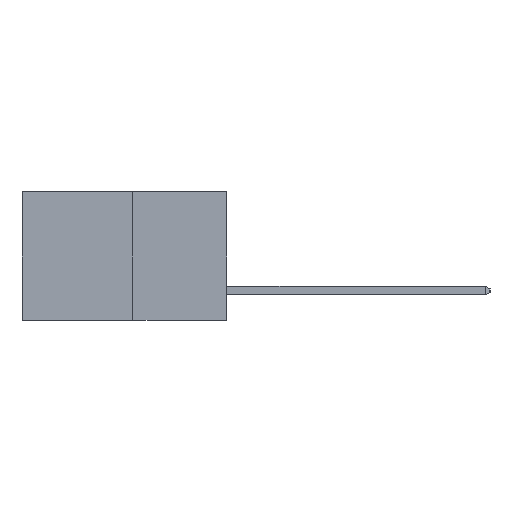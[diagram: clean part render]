
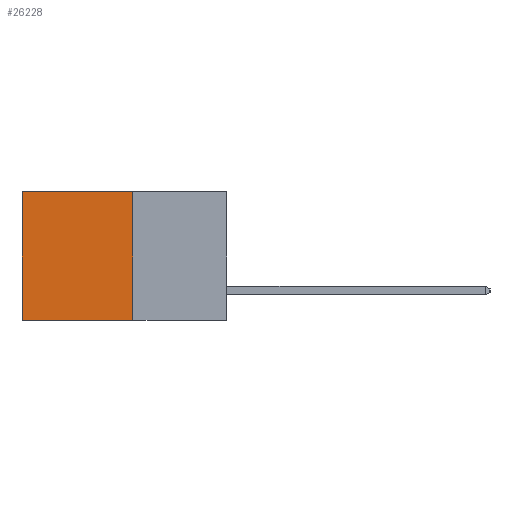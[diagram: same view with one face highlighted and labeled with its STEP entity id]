
A CAD part, left-side view. The second image highlights one B-rep face of the part: STEP entity #26228.
In plain terms, the highlighted planar face has unit normal (-1, 0, 0).
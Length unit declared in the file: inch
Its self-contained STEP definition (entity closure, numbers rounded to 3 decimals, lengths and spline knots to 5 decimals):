
#2866 = EDGE_CURVE ( 'NONE', #8837, #23938, #15441, .T. ) ;
#3015 = CARTESIAN_POINT ( 'NONE',  ( 0.277, 0.27, -0.37 ) ) ;
#3447 = ORIENTED_EDGE ( 'NONE', *, *, #18783, .T. ) ;
#6132 = ORIENTED_EDGE ( 'NONE', *, *, #12203, .F. ) ;
#6719 = ORIENTED_EDGE ( 'NONE', *, *, #9673, .T. ) ;
#6749 = AXIS2_PLACEMENT_3D ( 'NONE', #22543, #26654, #14082 ) ;
#6929 = VECTOR ( 'NONE', #21878, 39.37008 ) ;
#8186 = CARTESIAN_POINT ( 'NONE',  ( 0.277, 0.59, -0.37 ) ) ;
#8837 = VERTEX_POINT ( 'NONE', #9868 ) ;
#9673 = EDGE_CURVE ( 'NONE', #17967, #11888, #23120, .T. ) ;
#9868 = CARTESIAN_POINT ( 'NONE',  ( 0.277, 0.27, 0. ) ) ;
#11888 = VERTEX_POINT ( 'NONE', #14261 ) ;
#12203 = EDGE_CURVE ( 'NONE', #23938, #11888, #22958, .T. ) ;
#12469 = LINE ( 'NONE', #19770, #6929 ) ;
#12518 = VECTOR ( 'NONE', #20876, 39.37008 ) ;
#14082 = DIRECTION ( 'NONE',  ( 0., 0., -1. ) ) ;
#14261 = CARTESIAN_POINT ( 'NONE',  ( 0.277, 0.59, -0.37 ) ) ;
#15441 = LINE ( 'NONE', #18634, #20450 ) ;
#15634 = ORIENTED_EDGE ( 'NONE', *, *, #2866, .F. ) ;
#17905 = DIRECTION ( 'NONE',  ( 0., 1., 0. ) ) ;
#17967 = VERTEX_POINT ( 'NONE', #25047 ) ;
#18450 = DIRECTION ( 'NONE',  ( 0., 0., -1. ) ) ;
#18634 = CARTESIAN_POINT ( 'NONE',  ( 0.277, 0.27, -0.37 ) ) ;
#18783 = EDGE_CURVE ( 'NONE', #8837, #17967, #12469, .T. ) ;
#19770 = CARTESIAN_POINT ( 'NONE',  ( 0.277, 0.27, 0. ) ) ;
#20450 = VECTOR ( 'NONE', #18450, 39.37008 ) ;
#20876 = DIRECTION ( 'NONE',  ( 0., 0., -1. ) ) ;
#21686 = VECTOR ( 'NONE', #17905, 39.37008 ) ;
#21878 = DIRECTION ( 'NONE',  ( 0., 1., 0. ) ) ;
#22543 = CARTESIAN_POINT ( 'NONE',  ( 0.277, 0.27, -0.37 ) ) ;
#22958 = LINE ( 'NONE', #3015, #21686 ) ;
#23120 = LINE ( 'NONE', #8186, #12518 ) ;
#23938 = VERTEX_POINT ( 'NONE', #26784 ) ;
#24598 = PLANE ( 'NONE',  #6749 ) ;
#25047 = CARTESIAN_POINT ( 'NONE',  ( 0.277, 0.59, 0. ) ) ;
#25430 = EDGE_LOOP ( 'NONE', ( #6719, #6132, #15634, #3447 ) ) ;
#26228 = ADVANCED_FACE ( 'NONE', ( #27292 ), #24598, .F. ) ;
#26654 = DIRECTION ( 'NONE',  ( 1., 0., 0. ) ) ;
#26784 = CARTESIAN_POINT ( 'NONE',  ( 0.277, 0.27, -0.37 ) ) ;
#27292 = FACE_OUTER_BOUND ( 'NONE', #25430, .T. ) ;
